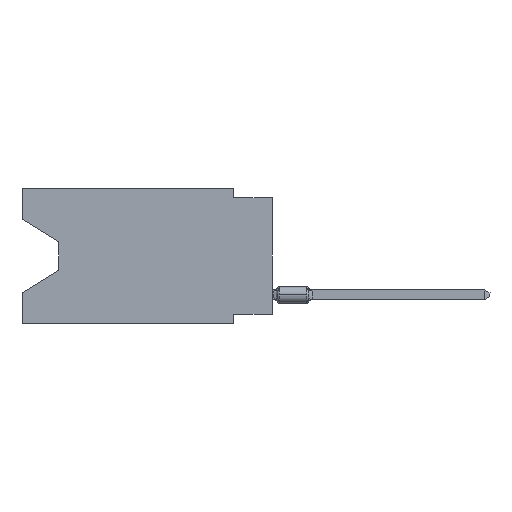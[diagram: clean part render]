
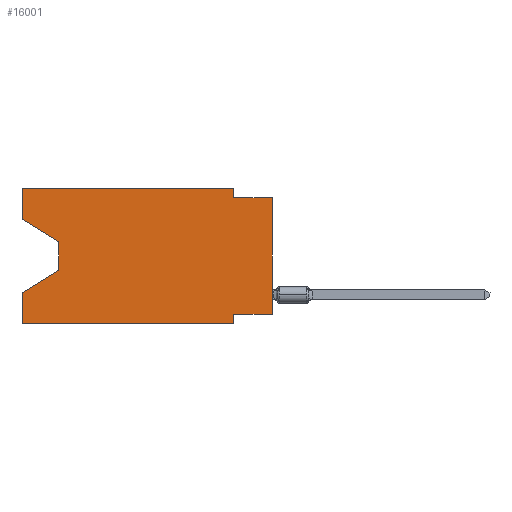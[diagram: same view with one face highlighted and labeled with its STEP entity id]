
A CAD part, left-side view. The second image highlights one B-rep face of the part: STEP entity #16001.
In plain terms, the highlighted planar face has unit normal (-1, 0, 0).
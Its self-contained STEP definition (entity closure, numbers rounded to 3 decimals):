
#269 = VECTOR ( 'NONE', #1427, 1000. ) ;
#302 = ORIENTED_EDGE ( 'NONE', *, *, #18172, .T. ) ;
#339 = VECTOR ( 'NONE', #14442, 1000. ) ;
#525 = DIRECTION ( 'NONE',  ( 0., -1., 0. ) ) ;
#630 = EDGE_CURVE ( 'NONE', #20656, #5941, #20689, .T. ) ;
#635 = ORIENTED_EDGE ( 'NONE', *, *, #8779, .F. ) ;
#752 = EDGE_CURVE ( 'NONE', #15699, #6534, #5138, .T. ) ;
#1083 = EDGE_CURVE ( 'NONE', #20656, #18419, #9881, .T. ) ;
#1427 = DIRECTION ( 'NONE',  ( 0., 1., 0. ) ) ;
#1492 = ORIENTED_EDGE ( 'NONE', *, *, #752, .T. ) ;
#1705 = VERTEX_POINT ( 'NONE', #8782 ) ;
#1747 = ORIENTED_EDGE ( 'NONE', *, *, #15229, .F. ) ;
#1920 = DIRECTION ( 'NONE',  ( 0., 0., 1. ) ) ;
#2106 = CARTESIAN_POINT ( 'NONE',  ( 0., 16.383, 0. ) ) ;
#2181 = VECTOR ( 'NONE', #3581, 1000. ) ;
#2386 = DIRECTION ( 'NONE',  ( 0., 0., -1. ) ) ;
#2419 = VECTOR ( 'NONE', #525, 1000. ) ;
#2857 = CARTESIAN_POINT ( 'NONE',  ( 0., 2.54, -8.89 ) ) ;
#2905 = LINE ( 'NONE', #16026, #14405 ) ;
#2995 = EDGE_CURVE ( 'NONE', #5941, #5302, #17201, .T. ) ;
#3581 = DIRECTION ( 'NONE',  ( 0., 0.855, -0.519 ) ) ;
#3937 = CARTESIAN_POINT ( 'NONE',  ( 0., 16.383, -2.038 ) ) ;
#4070 = VERTEX_POINT ( 'NONE', #10157 ) ;
#4305 = ORIENTED_EDGE ( 'NONE', *, *, #630, .F. ) ;
#4404 = VECTOR ( 'NONE', #8579, 1000. ) ;
#4791 = VECTOR ( 'NONE', #10542, 1000. ) ;
#4867 = EDGE_CURVE ( 'NONE', #13909, #12799, #14839, .T. ) ;
#5088 = CARTESIAN_POINT ( 'NONE',  ( 0., 0., -0.635 ) ) ;
#5138 = LINE ( 'NONE', #8724, #11074 ) ;
#5185 = ORIENTED_EDGE ( 'NONE', *, *, #7136, .T. ) ;
#5295 = CARTESIAN_POINT ( 'NONE',  ( 0., 16.383, -6.852 ) ) ;
#5302 = VERTEX_POINT ( 'NONE', #2857 ) ;
#5402 = EDGE_CURVE ( 'NONE', #15699, #1705, #8365, .T. ) ;
#5692 = VECTOR ( 'NONE', #6738, 1000. ) ;
#5941 = VERTEX_POINT ( 'NONE', #8965 ) ;
#6160 = CARTESIAN_POINT ( 'NONE',  ( 0., 13.97, -5.385 ) ) ;
#6534 = VERTEX_POINT ( 'NONE', #19298 ) ;
#6738 = DIRECTION ( 'NONE',  ( 0., 0., -1. ) ) ;
#6767 = ORIENTED_EDGE ( 'NONE', *, *, #16381, .T. ) ;
#6849 = CARTESIAN_POINT ( 'NONE',  ( 0., 2.54, 0. ) ) ;
#6898 = CARTESIAN_POINT ( 'NONE',  ( 0., 16.383, 0. ) ) ;
#6949 = ORIENTED_EDGE ( 'NONE', *, *, #10763, .F. ) ;
#7136 = EDGE_CURVE ( 'NONE', #6534, #15883, #19972, .T. ) ;
#7160 = LINE ( 'NONE', #6849, #5692 ) ;
#7674 = DIRECTION ( 'NONE',  ( 0., -1., 0. ) ) ;
#7910 = VECTOR ( 'NONE', #20367, 1000. ) ;
#8289 = VERTEX_POINT ( 'NONE', #11716 ) ;
#8319 = ORIENTED_EDGE ( 'NONE', *, *, #2995, .F. ) ;
#8365 = LINE ( 'NONE', #2106, #4404 ) ;
#8569 = LINE ( 'NONE', #14693, #2181 ) ;
#8579 = DIRECTION ( 'NONE',  ( 0., 0., 1. ) ) ;
#8602 = CARTESIAN_POINT ( 'NONE',  ( 0., 0., 0. ) ) ;
#8724 = CARTESIAN_POINT ( 'NONE',  ( 0., 16.383, -2.038 ) ) ;
#8779 = EDGE_CURVE ( 'NONE', #1705, #8289, #18358, .T. ) ;
#8782 = CARTESIAN_POINT ( 'NONE',  ( 0., 16.383, 0. ) ) ;
#8965 = CARTESIAN_POINT ( 'NONE',  ( 0., 2.54, -8.255 ) ) ;
#9881 = LINE ( 'NONE', #8602, #10084 ) ;
#10084 = VECTOR ( 'NONE', #1920, 1000. ) ;
#10157 = CARTESIAN_POINT ( 'NONE',  ( 0., 2.54, -0.635 ) ) ;
#10542 = DIRECTION ( 'NONE',  ( 0., 0., -1. ) ) ;
#10763 = EDGE_CURVE ( 'NONE', #4070, #18419, #16200, .T. ) ;
#10978 = AXIS2_PLACEMENT_3D ( 'NONE', #6898, #19796, #16412 ) ;
#11074 = VECTOR ( 'NONE', #11791, 1000. ) ;
#11716 = CARTESIAN_POINT ( 'NONE',  ( 0., 2.54, 0. ) ) ;
#11791 = DIRECTION ( 'NONE',  ( 0., -0.855, -0.519 ) ) ;
#11858 = PLANE ( 'NONE',  #10978 ) ;
#12126 = CARTESIAN_POINT ( 'NONE',  ( 0., 13.97, -3.505 ) ) ;
#12799 = VERTEX_POINT ( 'NONE', #5295 ) ;
#13071 = CARTESIAN_POINT ( 'NONE',  ( 0., 0., -8.255 ) ) ;
#13704 = EDGE_LOOP ( 'NONE', ( #1492, #5185, #6767, #19148, #302, #8319, #4305, #15059, #6949, #1747, #635, #13787 ) ) ;
#13787 = ORIENTED_EDGE ( 'NONE', *, *, #5402, .F. ) ;
#13909 = VERTEX_POINT ( 'NONE', #15389 ) ;
#14405 = VECTOR ( 'NONE', #7674, 1000. ) ;
#14442 = DIRECTION ( 'NONE',  ( 0., 0., 1. ) ) ;
#14693 = CARTESIAN_POINT ( 'NONE',  ( 0., 13.97, -5.385 ) ) ;
#14839 = LINE ( 'NONE', #16640, #339 ) ;
#15059 = ORIENTED_EDGE ( 'NONE', *, *, #1083, .T. ) ;
#15229 = EDGE_CURVE ( 'NONE', #8289, #4070, #7160, .T. ) ;
#15389 = CARTESIAN_POINT ( 'NONE',  ( 0., 16.383, -8.89 ) ) ;
#15699 = VERTEX_POINT ( 'NONE', #3937 ) ;
#15883 = VERTEX_POINT ( 'NONE', #6160 ) ;
#16001 = ADVANCED_FACE ( 'NONE', ( #16312 ), #11858, .F. ) ;
#16026 = CARTESIAN_POINT ( 'NONE',  ( 0., 16.383, -8.89 ) ) ;
#16200 = LINE ( 'NONE', #5088, #2419 ) ;
#16312 = FACE_OUTER_BOUND ( 'NONE', #13704, .T. ) ;
#16381 = EDGE_CURVE ( 'NONE', #15883, #12799, #8569, .T. ) ;
#16412 = DIRECTION ( 'NONE',  ( 0., 0., -1. ) ) ;
#16640 = CARTESIAN_POINT ( 'NONE',  ( 0., 16.383, 0. ) ) ;
#17086 = CARTESIAN_POINT ( 'NONE',  ( 0., 16.383, 0. ) ) ;
#17201 = LINE ( 'NONE', #18478, #4791 ) ;
#17494 = VECTOR ( 'NONE', #2386, 1000. ) ;
#18172 = EDGE_CURVE ( 'NONE', #13909, #5302, #2905, .T. ) ;
#18358 = LINE ( 'NONE', #17086, #7910 ) ;
#18419 = VERTEX_POINT ( 'NONE', #20846 ) ;
#18478 = CARTESIAN_POINT ( 'NONE',  ( 0., 2.54, -8.89 ) ) ;
#19148 = ORIENTED_EDGE ( 'NONE', *, *, #4867, .F. ) ;
#19161 = CARTESIAN_POINT ( 'NONE',  ( 0., 0., -8.255 ) ) ;
#19298 = CARTESIAN_POINT ( 'NONE',  ( 0., 13.97, -3.505 ) ) ;
#19796 = DIRECTION ( 'NONE',  ( 1., 0., 0. ) ) ;
#19972 = LINE ( 'NONE', #12126, #17494 ) ;
#20367 = DIRECTION ( 'NONE',  ( 0., -1., 0. ) ) ;
#20656 = VERTEX_POINT ( 'NONE', #19161 ) ;
#20689 = LINE ( 'NONE', #13071, #269 ) ;
#20846 = CARTESIAN_POINT ( 'NONE',  ( 0., 0., -0.635 ) ) ;
